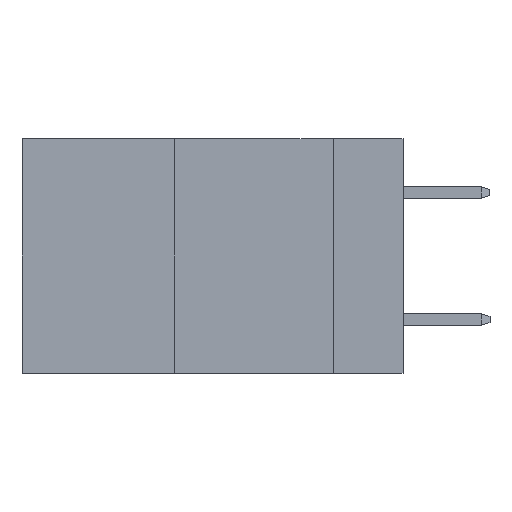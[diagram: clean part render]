
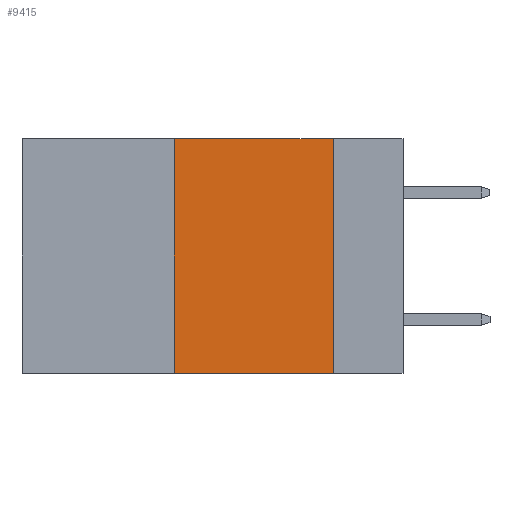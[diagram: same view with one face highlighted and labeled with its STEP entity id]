
A CAD part, left-side view. The second image highlights one B-rep face of the part: STEP entity #9415.
In plain terms, the highlighted planar face has unit normal (-1, 0, 0).
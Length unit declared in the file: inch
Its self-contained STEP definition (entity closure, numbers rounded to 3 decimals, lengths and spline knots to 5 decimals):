
#1899 = DIRECTION ( 'NONE',  ( 0., 0., -1. ) ) ;
#2137 = ORIENTED_EDGE ( 'NONE', *, *, #2273, .T. ) ;
#2273 = EDGE_CURVE ( 'NONE', #6202, #10072, #6526, .T. ) ;
#2586 = PLANE ( 'NONE',  #4690 ) ;
#2789 = EDGE_CURVE ( 'NONE', #6202, #3361, #4623, .T. ) ;
#3253 = EDGE_LOOP ( 'NONE', ( #8419, #10981, #5117, #2137 ) ) ;
#3361 = VERTEX_POINT ( 'NONE', #4213 ) ;
#3419 = CARTESIAN_POINT ( 'NONE',  ( 0., 0.6, 0. ) ) ;
#3710 = LINE ( 'NONE', #3419, #5894 ) ;
#4121 = CARTESIAN_POINT ( 'NONE',  ( 0., 0.11, 0. ) ) ;
#4142 = VECTOR ( 'NONE', #4283, 39.37008 ) ;
#4213 = CARTESIAN_POINT ( 'NONE',  ( 0., 0.36, 0. ) ) ;
#4283 = DIRECTION ( 'NONE',  ( 0., -1., 0. ) ) ;
#4623 = LINE ( 'NONE', #9027, #5121 ) ;
#4690 = AXIS2_PLACEMENT_3D ( 'NONE', #11446, #5990, #9378 ) ;
#5117 = ORIENTED_EDGE ( 'NONE', *, *, #2789, .F. ) ;
#5121 = VECTOR ( 'NONE', #10169, 39.37008 ) ;
#5894 = VECTOR ( 'NONE', #7833, 39.37008 ) ;
#5989 = VERTEX_POINT ( 'NONE', #4121 ) ;
#5990 = DIRECTION ( 'NONE',  ( 1., 0., 0. ) ) ;
#6202 = VERTEX_POINT ( 'NONE', #12451 ) ;
#6526 = LINE ( 'NONE', #12066, #4142 ) ;
#6675 = EDGE_CURVE ( 'NONE', #5989, #10072, #7392, .T. ) ;
#7241 = VECTOR ( 'NONE', #1899, 39.37008 ) ;
#7392 = LINE ( 'NONE', #11769, #7241 ) ;
#7833 = DIRECTION ( 'NONE',  ( 0., -1., 0. ) ) ;
#8419 = ORIENTED_EDGE ( 'NONE', *, *, #6675, .F. ) ;
#9027 = CARTESIAN_POINT ( 'NONE',  ( 0., 0.36, 0. ) ) ;
#9378 = DIRECTION ( 'NONE',  ( 0., 0., -1. ) ) ;
#9415 = ADVANCED_FACE ( 'NONE', ( #12655 ), #2586, .F. ) ;
#10072 = VERTEX_POINT ( 'NONE', #12055 ) ;
#10169 = DIRECTION ( 'NONE',  ( 0., 0., 1. ) ) ;
#10981 = ORIENTED_EDGE ( 'NONE', *, *, #11562, .F. ) ;
#11446 = CARTESIAN_POINT ( 'NONE',  ( 0., 0.6, 0. ) ) ;
#11562 = EDGE_CURVE ( 'NONE', #3361, #5989, #3710, .T. ) ;
#11769 = CARTESIAN_POINT ( 'NONE',  ( 0., 0.11, 0. ) ) ;
#12055 = CARTESIAN_POINT ( 'NONE',  ( 0., 0.11, -0.37 ) ) ;
#12066 = CARTESIAN_POINT ( 'NONE',  ( 0., 0.6, -0.37 ) ) ;
#12451 = CARTESIAN_POINT ( 'NONE',  ( 0., 0.36, -0.37 ) ) ;
#12655 = FACE_OUTER_BOUND ( 'NONE', #3253, .T. ) ;
